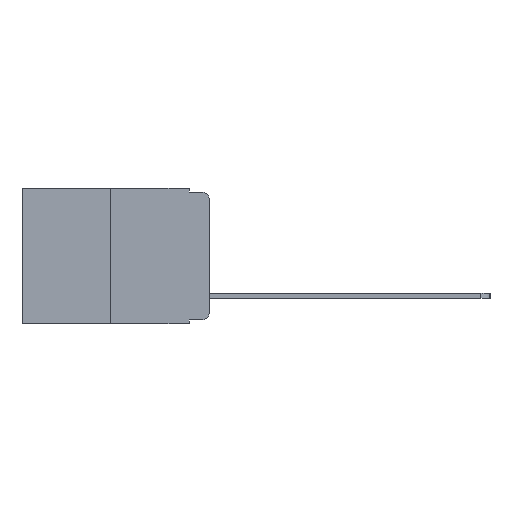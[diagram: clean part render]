
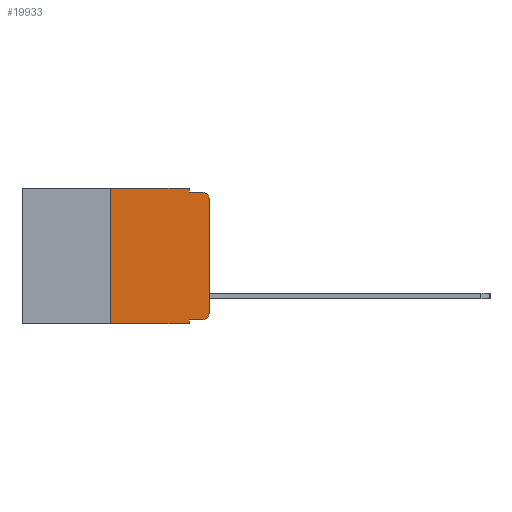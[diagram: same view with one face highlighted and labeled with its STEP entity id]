
A CAD part, left-side view. The second image highlights one B-rep face of the part: STEP entity #19933.
In plain terms, the highlighted planar face has unit normal (-1, 0, 0).
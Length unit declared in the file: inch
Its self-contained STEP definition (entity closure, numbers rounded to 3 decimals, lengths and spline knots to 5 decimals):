
#263 = CARTESIAN_POINT ( 'NONE',  ( 0., 0.051, -0.333 ) ) ;
#339 = DIRECTION ( 'NONE',  ( 1., 0., 0. ) ) ;
#1441 = CARTESIAN_POINT ( 'NONE',  ( 0., 0.473, -0.343 ) ) ;
#1577 = VERTEX_POINT ( 'NONE', #2701 ) ;
#1924 = EDGE_CURVE ( 'NONE', #5969, #24354, #12549, .T. ) ;
#2336 = CARTESIAN_POINT ( 'NONE',  ( 0., 0.473, 0. ) ) ;
#2701 = CARTESIAN_POINT ( 'NONE',  ( 0., 0.051, -0.343 ) ) ;
#2733 = VECTOR ( 'NONE', #7490, 39.37008 ) ;
#2783 = DIRECTION ( 'NONE',  ( -1., 0., 0. ) ) ;
#3404 = DIRECTION ( 'NONE',  ( 0., -1., 0. ) ) ;
#3657 = CIRCLE ( 'NONE', #22303, 0.02 ) ;
#3714 = CARTESIAN_POINT ( 'NONE',  ( 0., 0.051, 0. ) ) ;
#3953 = EDGE_CURVE ( 'NONE', #17623, #18160, #22921, .T. ) ;
#4059 = DIRECTION ( 'NONE',  ( 0., 0., -1. ) ) ;
#4166 = CARTESIAN_POINT ( 'NONE',  ( 0., 0.02, -0.313 ) ) ;
#4792 = DIRECTION ( 'NONE',  ( 0., 0., 1. ) ) ;
#5609 = EDGE_CURVE ( 'NONE', #20317, #1577, #25246, .T. ) ;
#5969 = VERTEX_POINT ( 'NONE', #9602 ) ;
#6165 = DIRECTION ( 'NONE',  ( 0., 0., -1. ) ) ;
#6517 = EDGE_CURVE ( 'NONE', #5969, #1577, #8003, .T. ) ;
#6572 = LINE ( 'NONE', #10713, #11869 ) ;
#6677 = AXIS2_PLACEMENT_3D ( 'NONE', #14759, #2783, #16807 ) ;
#6793 = ORIENTED_EDGE ( 'NONE', *, *, #11782, .T. ) ;
#7203 = VERTEX_POINT ( 'NONE', #10259 ) ;
#7239 = VECTOR ( 'NONE', #12550, 39.37008 ) ;
#7490 = DIRECTION ( 'NONE',  ( 0., -1., 0. ) ) ;
#8003 = LINE ( 'NONE', #1441, #2733 ) ;
#8032 = ORIENTED_EDGE ( 'NONE', *, *, #6517, .T. ) ;
#8145 = LINE ( 'NONE', #9289, #16990 ) ;
#9289 = CARTESIAN_POINT ( 'NONE',  ( 0., 0.473, 0. ) ) ;
#9330 = EDGE_CURVE ( 'NONE', #24354, #19124, #8145, .T. ) ;
#9602 = CARTESIAN_POINT ( 'NONE',  ( 0., 0.25, -0.343 ) ) ;
#9659 = ORIENTED_EDGE ( 'NONE', *, *, #3953, .F. ) ;
#9721 = CARTESIAN_POINT ( 'NONE',  ( 0., 0.25, 0. ) ) ;
#10105 = CARTESIAN_POINT ( 'NONE',  ( 0., 0., -0.313 ) ) ;
#10259 = CARTESIAN_POINT ( 'NONE',  ( 0., 0., -0.03 ) ) ;
#10518 = LINE ( 'NONE', #263, #20609 ) ;
#10713 = CARTESIAN_POINT ( 'NONE',  ( 0., 0., 0. ) ) ;
#10739 = ORIENTED_EDGE ( 'NONE', *, *, #9330, .F. ) ;
#11015 = EDGE_CURVE ( 'NONE', #19124, #17623, #20660, .T. ) ;
#11782 = EDGE_CURVE ( 'NONE', #20317, #12100, #10518, .T. ) ;
#11869 = VECTOR ( 'NONE', #4792, 39.37008 ) ;
#12100 = VERTEX_POINT ( 'NONE', #21373 ) ;
#12544 = EDGE_CURVE ( 'NONE', #12100, #23806, #3657, .T. ) ;
#12549 = LINE ( 'NONE', #13979, #7239 ) ;
#12550 = DIRECTION ( 'NONE',  ( 0., 0., 1. ) ) ;
#13264 = FACE_OUTER_BOUND ( 'NONE', #19854, .T. ) ;
#13979 = CARTESIAN_POINT ( 'NONE',  ( 0., 0.25, 0. ) ) ;
#14034 = VECTOR ( 'NONE', #19774, 39.37008 ) ;
#14035 = VECTOR ( 'NONE', #4059, 39.37008 ) ;
#14402 = DIRECTION ( 'NONE',  ( 0., 0., -1. ) ) ;
#14759 = CARTESIAN_POINT ( 'NONE',  ( 0., 0.02, -0.03 ) ) ;
#14965 = ORIENTED_EDGE ( 'NONE', *, *, #5609, .F. ) ;
#15110 = ORIENTED_EDGE ( 'NONE', *, *, #12544, .T. ) ;
#16774 = CARTESIAN_POINT ( 'NONE',  ( 0., 0.051, -0.01 ) ) ;
#16807 = DIRECTION ( 'NONE',  ( 0., 0., -1. ) ) ;
#16938 = DIRECTION ( 'NONE',  ( 0., -1., 0. ) ) ;
#16990 = VECTOR ( 'NONE', #3404, 39.37008 ) ;
#16991 = VECTOR ( 'NONE', #16938, 39.37008 ) ;
#17623 = VERTEX_POINT ( 'NONE', #16774 ) ;
#17746 = ORIENTED_EDGE ( 'NONE', *, *, #23991, .T. ) ;
#17749 = CARTESIAN_POINT ( 'NONE',  ( 0., 0.051, 0. ) ) ;
#18160 = VERTEX_POINT ( 'NONE', #22741 ) ;
#18198 = DIRECTION ( 'NONE',  ( -1., 0., 0. ) ) ;
#18418 = DIRECTION ( 'NONE',  ( 0., -1., 0. ) ) ;
#19082 = AXIS2_PLACEMENT_3D ( 'NONE', #2336, #339, #14402 ) ;
#19124 = VERTEX_POINT ( 'NONE', #3714 ) ;
#19602 = ORIENTED_EDGE ( 'NONE', *, *, #11015, .F. ) ;
#19774 = DIRECTION ( 'NONE',  ( 0., 0., -1. ) ) ;
#19854 = EDGE_LOOP ( 'NONE', ( #24377, #17746, #9659, #19602, #10739, #25702, #8032, #14965, #6793, #15110 ) ) ;
#19933 = ADVANCED_FACE ( 'NONE', ( #13264 ), #22390, .F. ) ;
#20317 = VERTEX_POINT ( 'NONE', #22038 ) ;
#20609 = VECTOR ( 'NONE', #18418, 39.37008 ) ;
#20660 = LINE ( 'NONE', #17749, #14034 ) ;
#21373 = CARTESIAN_POINT ( 'NONE',  ( 0., 0.02, -0.333 ) ) ;
#22038 = CARTESIAN_POINT ( 'NONE',  ( 0., 0.051, -0.333 ) ) ;
#22303 = AXIS2_PLACEMENT_3D ( 'NONE', #4166, #18198, #6165 ) ;
#22390 = PLANE ( 'NONE',  #19082 ) ;
#22741 = CARTESIAN_POINT ( 'NONE',  ( 0., 0.02, -0.01 ) ) ;
#22921 = LINE ( 'NONE', #24878, #16991 ) ;
#23198 = CIRCLE ( 'NONE', #6677, 0.02 ) ;
#23806 = VERTEX_POINT ( 'NONE', #10105 ) ;
#23991 = EDGE_CURVE ( 'NONE', #7203, #18160, #23198, .T. ) ;
#24023 = EDGE_CURVE ( 'NONE', #23806, #7203, #6572, .T. ) ;
#24354 = VERTEX_POINT ( 'NONE', #9721 ) ;
#24377 = ORIENTED_EDGE ( 'NONE', *, *, #24023, .T. ) ;
#24878 = CARTESIAN_POINT ( 'NONE',  ( 0., 0.051, -0.01 ) ) ;
#25246 = LINE ( 'NONE', #25912, #14035 ) ;
#25702 = ORIENTED_EDGE ( 'NONE', *, *, #1924, .F. ) ;
#25912 = CARTESIAN_POINT ( 'NONE',  ( 0., 0.051, 0. ) ) ;
